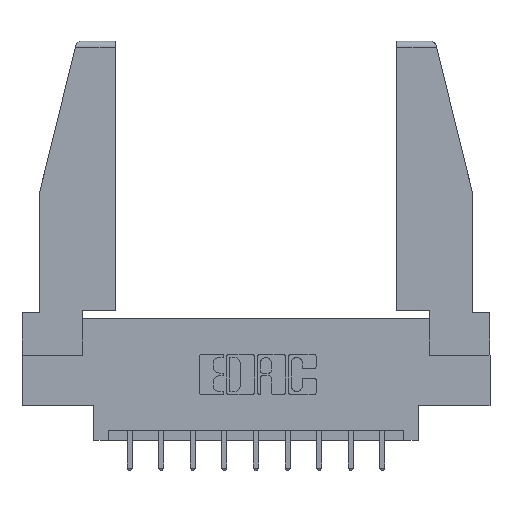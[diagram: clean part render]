
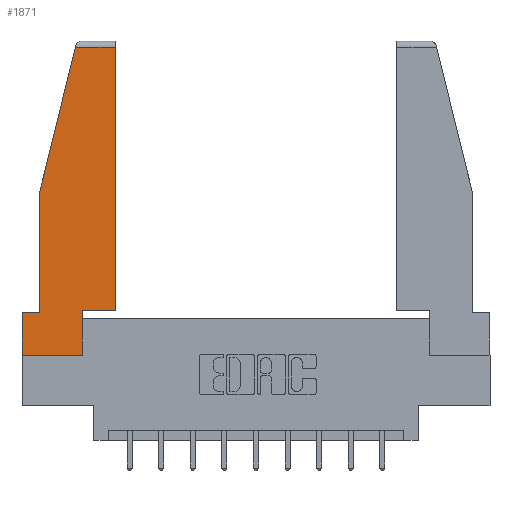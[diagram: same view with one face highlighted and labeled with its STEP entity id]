
A CAD part, top view. The second image highlights one B-rep face of the part: STEP entity #1871.
In plain terms, the highlighted planar face has unit normal (0, 0, 1).
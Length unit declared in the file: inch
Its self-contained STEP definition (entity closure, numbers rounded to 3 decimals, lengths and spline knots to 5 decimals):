
#162 = CARTESIAN_POINT ( 'NONE',  ( 0.271, 1.55, 0. ) ) ;
#298 = EDGE_CURVE ( 'NONE', #9662, #1346, #708, .T. ) ;
#302 = CARTESIAN_POINT ( 'NONE',  ( 0.297, 0.223, 0. ) ) ;
#555 = VECTOR ( 'NONE', #6751, 39.37008 ) ;
#708 = LINE ( 'NONE', #7515, #1733 ) ;
#729 = LINE ( 'NONE', #5711, #555 ) ;
#1011 = VECTOR ( 'NONE', #10955, 39.37008 ) ;
#1166 = VECTOR ( 'NONE', #12297, 39.37008 ) ;
#1346 = VERTEX_POINT ( 'NONE', #12701 ) ;
#1733 = VECTOR ( 'NONE', #9790, 39.37008 ) ;
#1777 = LINE ( 'NONE', #9506, #3287 ) ;
#1802 = VERTEX_POINT ( 'NONE', #13193 ) ;
#1834 = VERTEX_POINT ( 'NONE', #302 ) ;
#1871 = ADVANCED_FACE ( 'NONE', ( #7734 ), #2376, .T. ) ;
#1916 = EDGE_CURVE ( 'NONE', #6928, #3132, #4391, .T. ) ;
#2156 = ORIENTED_EDGE ( 'NONE', *, *, #4140, .T. ) ;
#2307 = CARTESIAN_POINT ( 'NONE',  ( 0.461, 0.223, 0. ) ) ;
#2376 = PLANE ( 'NONE',  #5070 ) ;
#2519 = CARTESIAN_POINT ( 'NONE',  ( 0., 0.21, 0. ) ) ;
#2575 = LINE ( 'NONE', #6835, #7961 ) ;
#2649 = VERTEX_POINT ( 'NONE', #2744 ) ;
#2744 = CARTESIAN_POINT ( 'NONE',  ( 0.2636, 1.52, 0. ) ) ;
#2967 = EDGE_CURVE ( 'NONE', #5215, #5309, #9079, .T. ) ;
#3075 = ORIENTED_EDGE ( 'NONE', *, *, #12654, .T. ) ;
#3132 = VERTEX_POINT ( 'NONE', #4676 ) ;
#3287 = VECTOR ( 'NONE', #13665, 39.37008 ) ;
#3672 = ORIENTED_EDGE ( 'NONE', *, *, #1916, .T. ) ;
#4140 = EDGE_CURVE ( 'NONE', #3132, #1802, #6181, .T. ) ;
#4158 = LINE ( 'NONE', #162, #10242 ) ;
#4391 = LINE ( 'NONE', #9863, #1011 ) ;
#4436 = CARTESIAN_POINT ( 'NONE',  ( 0.461, 1.52, 0. ) ) ;
#4569 = CARTESIAN_POINT ( 'NONE',  ( 0., 1.52, 0. ) ) ;
#4632 = DIRECTION ( 'NONE',  ( 0., 0., 1. ) ) ;
#4659 = EDGE_CURVE ( 'NONE', #5309, #2649, #7512, .T. ) ;
#4676 = CARTESIAN_POINT ( 'NONE',  ( 0.086, 0.21, 0. ) ) ;
#5070 = AXIS2_PLACEMENT_3D ( 'NONE', #9963, #4632, #12160 ) ;
#5166 = VECTOR ( 'NONE', #5765, 39.37008 ) ;
#5215 = VERTEX_POINT ( 'NONE', #9664 ) ;
#5309 = VERTEX_POINT ( 'NONE', #4436 ) ;
#5711 = CARTESIAN_POINT ( 'NONE',  ( 0.297, 0., 0. ) ) ;
#5765 = DIRECTION ( 'NONE',  ( -1., 0., 0. ) ) ;
#5862 = DIRECTION ( 'NONE',  ( 1., 0., 0. ) ) ;
#6181 = LINE ( 'NONE', #2519, #5166 ) ;
#6601 = DIRECTION ( 'NONE',  ( -1., 0., 0. ) ) ;
#6668 = DIRECTION ( 'NONE',  ( -0.239, -0.971, 0. ) ) ;
#6751 = DIRECTION ( 'NONE',  ( 0., 1., 0. ) ) ;
#6835 = CARTESIAN_POINT ( 'NONE',  ( 0.297, 0.223, 0. ) ) ;
#6928 = VERTEX_POINT ( 'NONE', #11641 ) ;
#7489 = EDGE_LOOP ( 'NONE', ( #13098, #12291, #9179, #3672, #2156, #12878, #8275, #3075, #13091 ) ) ;
#7512 = LINE ( 'NONE', #4569, #10044 ) ;
#7515 = CARTESIAN_POINT ( 'NONE',  ( 0., 0., 0. ) ) ;
#7706 = EDGE_CURVE ( 'NONE', #2649, #6928, #4158, .T. ) ;
#7734 = FACE_OUTER_BOUND ( 'NONE', #7489, .T. ) ;
#7961 = VECTOR ( 'NONE', #5862, 39.37008 ) ;
#8275 = ORIENTED_EDGE ( 'NONE', *, *, #298, .T. ) ;
#8431 = EDGE_CURVE ( 'NONE', #1802, #9662, #1777, .T. ) ;
#9079 = LINE ( 'NONE', #2307, #1166 ) ;
#9179 = ORIENTED_EDGE ( 'NONE', *, *, #7706, .T. ) ;
#9506 = CARTESIAN_POINT ( 'NONE',  ( 0., 0.21, 0. ) ) ;
#9662 = VERTEX_POINT ( 'NONE', #12661 ) ;
#9664 = CARTESIAN_POINT ( 'NONE',  ( 0.461, 0.223, 0. ) ) ;
#9790 = DIRECTION ( 'NONE',  ( 1., 0., 0. ) ) ;
#9863 = CARTESIAN_POINT ( 'NONE',  ( 0.086, 0.8, 0. ) ) ;
#9963 = CARTESIAN_POINT ( 'NONE',  ( 0., 0., 0. ) ) ;
#9969 = EDGE_CURVE ( 'NONE', #1834, #5215, #2575, .T. ) ;
#10044 = VECTOR ( 'NONE', #6601, 39.37008 ) ;
#10242 = VECTOR ( 'NONE', #6668, 39.37008 ) ;
#10955 = DIRECTION ( 'NONE',  ( 0., -1., 0. ) ) ;
#11641 = CARTESIAN_POINT ( 'NONE',  ( 0.086, 0.8, 0. ) ) ;
#12160 = DIRECTION ( 'NONE',  ( 1., 0., 0. ) ) ;
#12291 = ORIENTED_EDGE ( 'NONE', *, *, #4659, .T. ) ;
#12297 = DIRECTION ( 'NONE',  ( 0., 1., 0. ) ) ;
#12654 = EDGE_CURVE ( 'NONE', #1346, #1834, #729, .T. ) ;
#12661 = CARTESIAN_POINT ( 'NONE',  ( 0., 0., 0. ) ) ;
#12701 = CARTESIAN_POINT ( 'NONE',  ( 0.297, 0., 0. ) ) ;
#12878 = ORIENTED_EDGE ( 'NONE', *, *, #8431, .T. ) ;
#13091 = ORIENTED_EDGE ( 'NONE', *, *, #9969, .T. ) ;
#13098 = ORIENTED_EDGE ( 'NONE', *, *, #2967, .T. ) ;
#13193 = CARTESIAN_POINT ( 'NONE',  ( 0., 0.21, 0. ) ) ;
#13665 = DIRECTION ( 'NONE',  ( 0., -1., 0. ) ) ;
